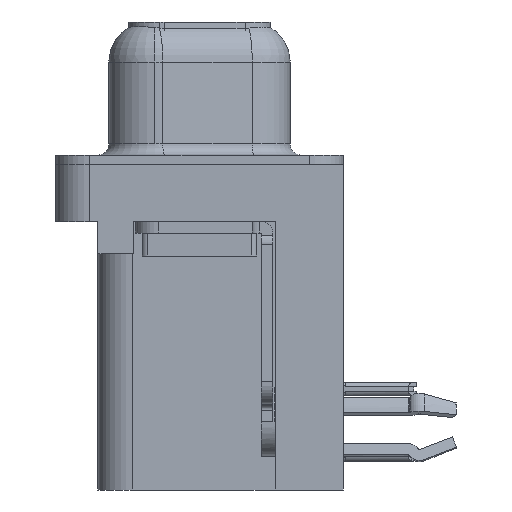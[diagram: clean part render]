
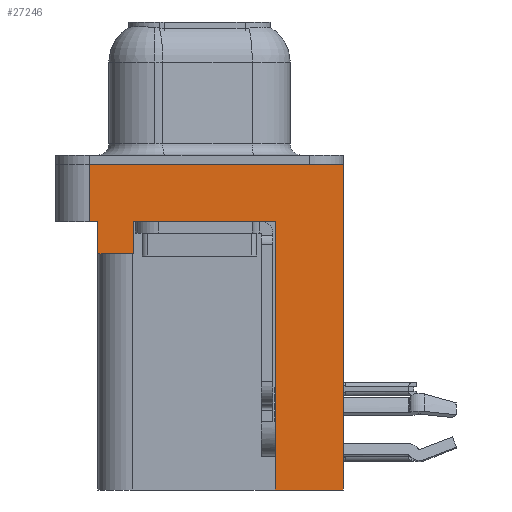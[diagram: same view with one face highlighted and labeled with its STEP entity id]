
A CAD part, left-side view. The second image highlights one B-rep face of the part: STEP entity #27246.
In plain terms, the highlighted planar face has unit normal (-1, 0, 0).
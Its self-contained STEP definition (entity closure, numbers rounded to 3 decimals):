
#426 = VECTOR ( 'NONE', #8716, 1000. ) ;
#615 = VERTEX_POINT ( 'NONE', #22604 ) ;
#690 = ORIENTED_EDGE ( 'NONE', *, *, #15079, .T. ) ;
#1238 = LINE ( 'NONE', #18988, #25806 ) ;
#1493 = VECTOR ( 'NONE', #13546, 1000. ) ;
#1498 = LINE ( 'NONE', #25853, #5632 ) ;
#1608 = CARTESIAN_POINT ( 'NONE',  ( -2.935, 2.895, -3.9 ) ) ;
#2235 = VERTEX_POINT ( 'NONE', #16662 ) ;
#2677 = FACE_OUTER_BOUND ( 'NONE', #23598, .T. ) ;
#2684 = CARTESIAN_POINT ( 'NONE',  ( -2.935, 4.775, -2.5 ) ) ;
#2733 = EDGE_CURVE ( 'NONE', #15537, #14295, #28042, .T. ) ;
#2794 = LINE ( 'NONE', #22429, #1493 ) ;
#3748 = AXIS2_PLACEMENT_3D ( 'NONE', #8851, #11430, #20165 ) ;
#3749 = CARTESIAN_POINT ( 'NONE',  ( -2.935, -3.295, -14.2 ) ) ;
#3877 = EDGE_CURVE ( 'NONE', #2235, #615, #7982, .T. ) ;
#3927 = CARTESIAN_POINT ( 'NONE',  ( -2.935, 4.775, 0. ) ) ;
#4112 = EDGE_CURVE ( 'NONE', #24109, #615, #10920, .T. ) ;
#4840 = EDGE_CURVE ( 'NONE', #11765, #16743, #10848, .T. ) ;
#5352 = CARTESIAN_POINT ( 'NONE',  ( -2.935, -6.275, 0. ) ) ;
#5632 = VECTOR ( 'NONE', #5799, 1000. ) ;
#5799 = DIRECTION ( 'NONE',  ( 0., -1., 0. ) ) ;
#6128 = EDGE_CURVE ( 'NONE', #27868, #14295, #1498, .T. ) ;
#6376 = VECTOR ( 'NONE', #25701, 1000. ) ;
#6721 = ORIENTED_EDGE ( 'NONE', *, *, #23347, .F. ) ;
#6763 = VERTEX_POINT ( 'NONE', #23145 ) ;
#6854 = LINE ( 'NONE', #2684, #11358 ) ;
#7077 = ORIENTED_EDGE ( 'NONE', *, *, #27681, .F. ) ;
#7982 = LINE ( 'NONE', #16710, #18198 ) ;
#8716 = DIRECTION ( 'NONE',  ( 0., 0., 1. ) ) ;
#8851 = CARTESIAN_POINT ( 'NONE',  ( -2.935, -6.275, -2.5 ) ) ;
#9196 = ORIENTED_EDGE ( 'NONE', *, *, #15025, .F. ) ;
#10353 = DIRECTION ( 'NONE',  ( 0., 0., 1. ) ) ;
#10441 = CARTESIAN_POINT ( 'NONE',  ( -2.935, 4.425, -3.9 ) ) ;
#10848 = LINE ( 'NONE', #26166, #16683 ) ;
#10920 = LINE ( 'NONE', #3749, #20968 ) ;
#11291 = DIRECTION ( 'NONE',  ( 0., 0., 1. ) ) ;
#11358 = VECTOR ( 'NONE', #11291, 1000. ) ;
#11430 = DIRECTION ( 'NONE',  ( -1., 0., 0. ) ) ;
#11570 = PLANE ( 'NONE',  #3748 ) ;
#11685 = CARTESIAN_POINT ( 'NONE',  ( -2.935, 4.425, -3.9 ) ) ;
#11765 = VERTEX_POINT ( 'NONE', #3927 ) ;
#13374 = CARTESIAN_POINT ( 'NONE',  ( -2.935, 4.775, -2.5 ) ) ;
#13546 = DIRECTION ( 'NONE',  ( 0., 1., 0. ) ) ;
#13803 = CARTESIAN_POINT ( 'NONE',  ( -2.935, 4.425, -2.5 ) ) ;
#14120 = ORIENTED_EDGE ( 'NONE', *, *, #6128, .T. ) ;
#14295 = VERTEX_POINT ( 'NONE', #13803 ) ;
#14307 = VERTEX_POINT ( 'NONE', #27107 ) ;
#15025 = EDGE_CURVE ( 'NONE', #27868, #11765, #6854, .T. ) ;
#15079 = EDGE_CURVE ( 'NONE', #14307, #16743, #1238, .T. ) ;
#15537 = VERTEX_POINT ( 'NONE', #11685 ) ;
#16016 = ORIENTED_EDGE ( 'NONE', *, *, #4840, .F. ) ;
#16662 = CARTESIAN_POINT ( 'NONE',  ( -2.935, 2.895, -2.5 ) ) ;
#16683 = VECTOR ( 'NONE', #24453, 1000. ) ;
#16710 = CARTESIAN_POINT ( 'NONE',  ( -2.935, -6.275, -2.5 ) ) ;
#16743 = VERTEX_POINT ( 'NONE', #5352 ) ;
#17236 = LINE ( 'NONE', #19100, #6376 ) ;
#18091 = ORIENTED_EDGE ( 'NONE', *, *, #4112, .F. ) ;
#18198 = VECTOR ( 'NONE', #23745, 1000. ) ;
#18988 = CARTESIAN_POINT ( 'NONE',  ( -2.935, -6.275, -2.5 ) ) ;
#19100 = CARTESIAN_POINT ( 'NONE',  ( -2.935, -3.295, -14.2 ) ) ;
#19103 = EDGE_CURVE ( 'NONE', #6763, #2235, #21241, .T. ) ;
#20165 = DIRECTION ( 'NONE',  ( 0., 0., 1. ) ) ;
#20742 = DIRECTION ( 'NONE',  ( 0., 0., 1. ) ) ;
#20968 = VECTOR ( 'NONE', #21229, 1000. ) ;
#21229 = DIRECTION ( 'NONE',  ( 0., 0., 1. ) ) ;
#21241 = LINE ( 'NONE', #1608, #27357 ) ;
#22154 = ORIENTED_EDGE ( 'NONE', *, *, #19103, .T. ) ;
#22429 = CARTESIAN_POINT ( 'NONE',  ( -2.935, 4.425, -3.9 ) ) ;
#22604 = CARTESIAN_POINT ( 'NONE',  ( -2.935, -3.295, -2.5 ) ) ;
#23145 = CARTESIAN_POINT ( 'NONE',  ( -2.935, 2.895, -3.9 ) ) ;
#23347 = EDGE_CURVE ( 'NONE', #14307, #24109, #17236, .T. ) ;
#23598 = EDGE_LOOP ( 'NONE', ( #16016, #9196, #14120, #28114, #7077, #22154, #28052, #18091, #6721, #690 ) ) ;
#23745 = DIRECTION ( 'NONE',  ( 0., -1., 0. ) ) ;
#24018 = CARTESIAN_POINT ( 'NONE',  ( -2.935, -3.295, -14.2 ) ) ;
#24109 = VERTEX_POINT ( 'NONE', #24018 ) ;
#24453 = DIRECTION ( 'NONE',  ( 0., -1., 0. ) ) ;
#25701 = DIRECTION ( 'NONE',  ( 0., 1., 0. ) ) ;
#25806 = VECTOR ( 'NONE', #20742, 1000. ) ;
#25853 = CARTESIAN_POINT ( 'NONE',  ( -2.935, -6.275, -2.5 ) ) ;
#26166 = CARTESIAN_POINT ( 'NONE',  ( -2.935, -6.275, 0. ) ) ;
#27107 = CARTESIAN_POINT ( 'NONE',  ( -2.935, -6.275, -14.2 ) ) ;
#27246 = ADVANCED_FACE ( 'NONE', ( #2677 ), #11570, .T. ) ;
#27357 = VECTOR ( 'NONE', #10353, 1000. ) ;
#27681 = EDGE_CURVE ( 'NONE', #6763, #15537, #2794, .T. ) ;
#27868 = VERTEX_POINT ( 'NONE', #13374 ) ;
#28042 = LINE ( 'NONE', #10441, #426 ) ;
#28052 = ORIENTED_EDGE ( 'NONE', *, *, #3877, .T. ) ;
#28114 = ORIENTED_EDGE ( 'NONE', *, *, #2733, .F. ) ;
